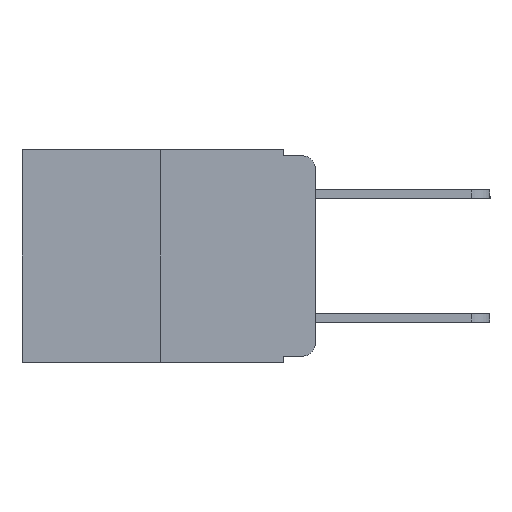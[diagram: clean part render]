
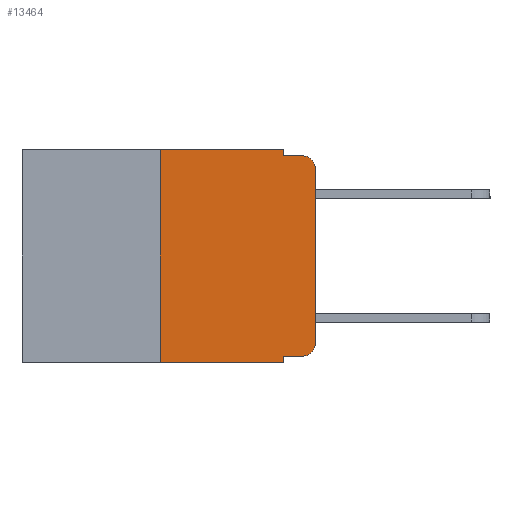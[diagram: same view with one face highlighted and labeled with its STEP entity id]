
A CAD part, left-side view. The second image highlights one B-rep face of the part: STEP entity #13464.
In plain terms, the highlighted planar face has unit normal (-1, 0, 0).
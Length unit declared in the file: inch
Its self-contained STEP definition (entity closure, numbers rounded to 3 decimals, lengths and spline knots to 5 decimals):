
#611 = CARTESIAN_POINT ( 'NONE',  ( 0., 0.051, -0.333 ) ) ;
#907 = CARTESIAN_POINT ( 'NONE',  ( 0., 0.473, -0.343 ) ) ;
#1047 = DIRECTION ( 'NONE',  ( 0., -1., 0. ) ) ;
#1141 = DIRECTION ( 'NONE',  ( 0., 0., -1. ) ) ;
#1370 = DIRECTION ( 'NONE',  ( 0., 0., -1. ) ) ;
#1426 = VERTEX_POINT ( 'NONE', #2934 ) ;
#1633 = LINE ( 'NONE', #21776, #5587 ) ;
#1917 = EDGE_CURVE ( 'NONE', #17759, #1426, #7698, .T. ) ;
#2315 = DIRECTION ( 'NONE',  ( 0., -1., 0. ) ) ;
#2531 = LINE ( 'NONE', #11846, #20132 ) ;
#2765 = EDGE_CURVE ( 'NONE', #6167, #12506, #6056, .T. ) ;
#2934 = CARTESIAN_POINT ( 'NONE',  ( 0., 0.02, -0.01 ) ) ;
#3057 = DIRECTION ( 'NONE',  ( 0., 0., 1. ) ) ;
#3179 = DIRECTION ( 'NONE',  ( 0., 0., -1. ) ) ;
#3924 = ORIENTED_EDGE ( 'NONE', *, *, #4860, .F. ) ;
#4187 = VECTOR ( 'NONE', #1047, 39.37008 ) ;
#4462 = EDGE_LOOP ( 'NONE', ( #20250, #8538, #5289, #13540, #12765, #3924, #11168, #13047, #11187, #5806 ) ) ;
#4520 = CARTESIAN_POINT ( 'NONE',  ( 0., 0.02, -0.333 ) ) ;
#4712 = LINE ( 'NONE', #907, #4187 ) ;
#4737 = CARTESIAN_POINT ( 'NONE',  ( 0., 0., 0. ) ) ;
#4860 = EDGE_CURVE ( 'NONE', #19631, #6167, #2531, .T. ) ;
#4867 = CARTESIAN_POINT ( 'NONE',  ( 0., 0.051, 0. ) ) ;
#5289 = ORIENTED_EDGE ( 'NONE', *, *, #1917, .F. ) ;
#5531 = CARTESIAN_POINT ( 'NONE',  ( 0., 0.051, -0.01 ) ) ;
#5587 = VECTOR ( 'NONE', #1370, 39.37008 ) ;
#5806 = ORIENTED_EDGE ( 'NONE', *, *, #16775, .T. ) ;
#5848 = AXIS2_PLACEMENT_3D ( 'NONE', #7413, #19357, #9147 ) ;
#5949 = PLANE ( 'NONE',  #11261 ) ;
#6015 = LINE ( 'NONE', #611, #8460 ) ;
#6025 = EDGE_CURVE ( 'NONE', #14558, #10409, #8054, .T. ) ;
#6056 = LINE ( 'NONE', #18211, #14105 ) ;
#6167 = VERTEX_POINT ( 'NONE', #20423 ) ;
#6289 = CARTESIAN_POINT ( 'NONE',  ( 0., 0.051, -0.333 ) ) ;
#7413 = CARTESIAN_POINT ( 'NONE',  ( 0., 0.02, -0.03 ) ) ;
#7698 = LINE ( 'NONE', #5531, #11710 ) ;
#8054 = LINE ( 'NONE', #4737, #20570 ) ;
#8061 = EDGE_CURVE ( 'NONE', #21238, #16510, #21800, .T. ) ;
#8168 = CIRCLE ( 'NONE', #20501, 0.02 ) ;
#8319 = EDGE_CURVE ( 'NONE', #10409, #1426, #16517, .T. ) ;
#8460 = VECTOR ( 'NONE', #2315, 39.37008 ) ;
#8538 = ORIENTED_EDGE ( 'NONE', *, *, #8319, .T. ) ;
#8870 = CARTESIAN_POINT ( 'NONE',  ( 0., 0.051, -0.01 ) ) ;
#9147 = DIRECTION ( 'NONE',  ( 0., 0., -1. ) ) ;
#9174 = EDGE_CURVE ( 'NONE', #19631, #16510, #4712, .T. ) ;
#9422 = DIRECTION ( 'NONE',  ( 1., 0., 0. ) ) ;
#10157 = CARTESIAN_POINT ( 'NONE',  ( 0., 0.25, -0.343 ) ) ;
#10177 = DIRECTION ( 'NONE',  ( 0., 0., 1. ) ) ;
#10409 = VERTEX_POINT ( 'NONE', #11520 ) ;
#11027 = VERTEX_POINT ( 'NONE', #4520 ) ;
#11168 = ORIENTED_EDGE ( 'NONE', *, *, #9174, .T. ) ;
#11187 = ORIENTED_EDGE ( 'NONE', *, *, #15374, .T. ) ;
#11226 = FACE_OUTER_BOUND ( 'NONE', #4462, .T. ) ;
#11261 = AXIS2_PLACEMENT_3D ( 'NONE', #12794, #9422, #21309 ) ;
#11383 = DIRECTION ( 'NONE',  ( -1., 0., 0. ) ) ;
#11520 = CARTESIAN_POINT ( 'NONE',  ( 0., 0., -0.03 ) ) ;
#11710 = VECTOR ( 'NONE', #14251, 39.37008 ) ;
#11846 = CARTESIAN_POINT ( 'NONE',  ( 0., 0.25, 0. ) ) ;
#12353 = CARTESIAN_POINT ( 'NONE',  ( 0., 0.051, -0.343 ) ) ;
#12506 = VERTEX_POINT ( 'NONE', #18698 ) ;
#12765 = ORIENTED_EDGE ( 'NONE', *, *, #2765, .F. ) ;
#12794 = CARTESIAN_POINT ( 'NONE',  ( 0., 0.473, 0. ) ) ;
#13047 = ORIENTED_EDGE ( 'NONE', *, *, #8061, .F. ) ;
#13464 = ADVANCED_FACE ( 'NONE', ( #11226 ), #5949, .F. ) ;
#13540 = ORIENTED_EDGE ( 'NONE', *, *, #19484, .F. ) ;
#14105 = VECTOR ( 'NONE', #20806, 39.37008 ) ;
#14251 = DIRECTION ( 'NONE',  ( 0., -1., 0. ) ) ;
#14314 = CARTESIAN_POINT ( 'NONE',  ( 0., 0., -0.313 ) ) ;
#14558 = VERTEX_POINT ( 'NONE', #14314 ) ;
#15374 = EDGE_CURVE ( 'NONE', #21238, #11027, #6015, .T. ) ;
#16510 = VERTEX_POINT ( 'NONE', #12353 ) ;
#16517 = CIRCLE ( 'NONE', #5848, 0.02 ) ;
#16775 = EDGE_CURVE ( 'NONE', #11027, #14558, #8168, .T. ) ;
#17318 = VECTOR ( 'NONE', #3179, 39.37008 ) ;
#17759 = VERTEX_POINT ( 'NONE', #8870 ) ;
#18211 = CARTESIAN_POINT ( 'NONE',  ( 0., 0.473, 0. ) ) ;
#18698 = CARTESIAN_POINT ( 'NONE',  ( 0., 0.051, 0. ) ) ;
#19357 = DIRECTION ( 'NONE',  ( -1., 0., 0. ) ) ;
#19484 = EDGE_CURVE ( 'NONE', #12506, #17759, #1633, .T. ) ;
#19631 = VERTEX_POINT ( 'NONE', #10157 ) ;
#20132 = VECTOR ( 'NONE', #10177, 39.37008 ) ;
#20250 = ORIENTED_EDGE ( 'NONE', *, *, #6025, .T. ) ;
#20423 = CARTESIAN_POINT ( 'NONE',  ( 0., 0.25, 0. ) ) ;
#20501 = AXIS2_PLACEMENT_3D ( 'NONE', #21530, #11383, #1141 ) ;
#20570 = VECTOR ( 'NONE', #3057, 39.37008 ) ;
#20806 = DIRECTION ( 'NONE',  ( 0., -1., 0. ) ) ;
#21238 = VERTEX_POINT ( 'NONE', #6289 ) ;
#21309 = DIRECTION ( 'NONE',  ( 0., 0., -1. ) ) ;
#21530 = CARTESIAN_POINT ( 'NONE',  ( 0., 0.02, -0.313 ) ) ;
#21776 = CARTESIAN_POINT ( 'NONE',  ( 0., 0.051, 0. ) ) ;
#21800 = LINE ( 'NONE', #4867, #17318 ) ;
